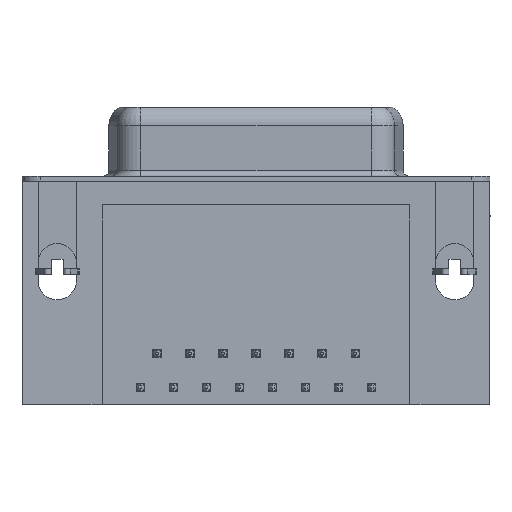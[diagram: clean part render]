
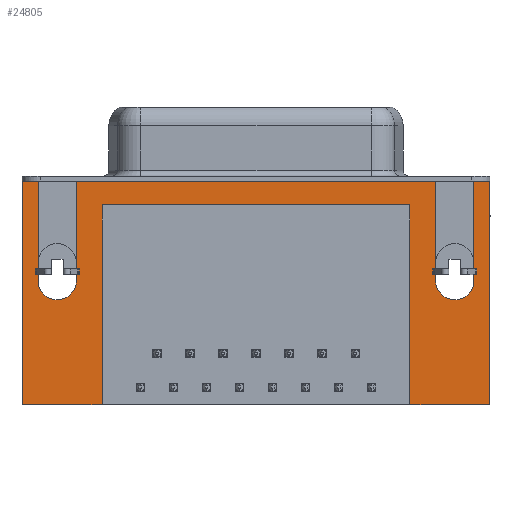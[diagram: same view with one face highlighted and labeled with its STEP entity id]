
A CAD part, front view. The second image highlights one B-rep face of the part: STEP entity #24805.
In plain terms, the highlighted planar face has unit normal (0, -1, 0).
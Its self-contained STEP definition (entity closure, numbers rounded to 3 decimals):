
#329 = CARTESIAN_POINT ( 'NONE',  ( -2.935, -6.275, 0. ) ) ;
#400 = VERTEX_POINT ( 'NONE', #22086 ) ;
#438 = ORIENTED_EDGE ( 'NONE', *, *, #1321, .F. ) ;
#682 = ORIENTED_EDGE ( 'NONE', *, *, #13333, .F. ) ;
#799 = CARTESIAN_POINT ( 'NONE',  ( -2.935, -6.275, 0. ) ) ;
#941 = FACE_OUTER_BOUND ( 'NONE', #15369, .T. ) ;
#1094 = CARTESIAN_POINT ( 'NONE',  ( 29.555, -6.275, -2. ) ) ;
#1101 = ORIENTED_EDGE ( 'NONE', *, *, #20498, .F. ) ;
#1321 = EDGE_CURVE ( 'NONE', #11784, #4898, #9651, .T. ) ;
#1620 = EDGE_CURVE ( 'NONE', #22914, #3859, #9228, .T. ) ;
#1792 = CARTESIAN_POINT ( 'NONE',  ( 3.765, -6.275, -2. ) ) ;
#1860 = DIRECTION ( 'NONE',  ( 0., 0., 1. ) ) ;
#2117 = DIRECTION ( 'NONE',  ( 0., 0., 1. ) ) ;
#2202 = DIRECTION ( 'NONE',  ( -1., 0., 0. ) ) ;
#2442 = CARTESIAN_POINT ( 'NONE',  ( 34.92, -6.275, 0. ) ) ;
#3032 = DIRECTION ( 'NONE',  ( 0., 0., -1. ) ) ;
#3361 = CARTESIAN_POINT ( 'NONE',  ( 31.72, -6.275, -8.35 ) ) ;
#3405 = DIRECTION ( 'NONE',  ( -1., 0., 0. ) ) ;
#3544 = EDGE_CURVE ( 'NONE', #16267, #22914, #26821, .T. ) ;
#3791 = CARTESIAN_POINT ( 'NONE',  ( 3.765, -6.275, -2. ) ) ;
#3859 = VERTEX_POINT ( 'NONE', #20307 ) ;
#3900 = DIRECTION ( 'NONE',  ( 0., 0., -1. ) ) ;
#4011 = CARTESIAN_POINT ( 'NONE',  ( 36.255, -6.275, -18.76 ) ) ;
#4176 = ORIENTED_EDGE ( 'NONE', *, *, #25894, .F. ) ;
#4520 = CARTESIAN_POINT ( 'NONE',  ( -1.6, -6.275, 0. ) ) ;
#4898 = VERTEX_POINT ( 'NONE', #5976 ) ;
#5200 = VERTEX_POINT ( 'NONE', #15408 ) ;
#5457 = EDGE_CURVE ( 'NONE', #5200, #16267, #13866, .T. ) ;
#5460 = VECTOR ( 'NONE', #7356, 1000. ) ;
#5506 = LINE ( 'NONE', #25995, #5460 ) ;
#5624 = ORIENTED_EDGE ( 'NONE', *, *, #1620, .F. ) ;
#5661 = VECTOR ( 'NONE', #3900, 1000. ) ;
#5976 = CARTESIAN_POINT ( 'NONE',  ( 1.6, -6.275, -8.35 ) ) ;
#6166 = CARTESIAN_POINT ( 'NONE',  ( 33.32, -6.275, -8.35 ) ) ;
#6206 = CARTESIAN_POINT ( 'NONE',  ( -2.935, -6.275, -2.5 ) ) ;
#6338 = VERTEX_POINT ( 'NONE', #4520 ) ;
#6771 = VECTOR ( 'NONE', #2117, 1000. ) ;
#6832 = EDGE_CURVE ( 'NONE', #4898, #24141, #6899, .T. ) ;
#6899 = LINE ( 'NONE', #18880, #6771 ) ;
#7152 = DIRECTION ( 'NONE',  ( 0., 0., 1. ) ) ;
#7177 = EDGE_CURVE ( 'NONE', #6338, #11784, #5506, .T. ) ;
#7356 = DIRECTION ( 'NONE',  ( 0., 0., -1. ) ) ;
#7525 = CARTESIAN_POINT ( 'NONE',  ( -2.935, -6.275, 0. ) ) ;
#7764 = CARTESIAN_POINT ( 'NONE',  ( -2.935, -6.275, -18.76 ) ) ;
#7915 = VECTOR ( 'NONE', #7152, 1000. ) ;
#8144 = ORIENTED_EDGE ( 'NONE', *, *, #9149, .F. ) ;
#8220 = LINE ( 'NONE', #11351, #7915 ) ;
#8268 = LINE ( 'NONE', #1792, #5661 ) ;
#8271 = DIRECTION ( 'NONE',  ( -1., 0., 0. ) ) ;
#8282 = ORIENTED_EDGE ( 'NONE', *, *, #5457, .F. ) ;
#8578 = VERTEX_POINT ( 'NONE', #12270 ) ;
#8662 = VERTEX_POINT ( 'NONE', #21041 ) ;
#8749 = VECTOR ( 'NONE', #1860, 1000. ) ;
#9149 = EDGE_CURVE ( 'NONE', #8662, #21470, #17370, .T. ) ;
#9228 = LINE ( 'NONE', #2442, #8749 ) ;
#9538 = VERTEX_POINT ( 'NONE', #4011 ) ;
#9651 = CIRCLE ( 'NONE', #10588, 1.6 ) ;
#9961 = ORIENTED_EDGE ( 'NONE', *, *, #7177, .F. ) ;
#10121 = ORIENTED_EDGE ( 'NONE', *, *, #11027, .F. ) ;
#10528 = EDGE_CURVE ( 'NONE', #16857, #8662, #8268, .T. ) ;
#10588 = AXIS2_PLACEMENT_3D ( 'NONE', #11688, #11680, #11626 ) ;
#11027 = EDGE_CURVE ( 'NONE', #8578, #16857, #26663, .T. ) ;
#11095 = EDGE_CURVE ( 'NONE', #3859, #400, #26489, .T. ) ;
#11351 = CARTESIAN_POINT ( 'NONE',  ( 36.255, -6.275, -2.5 ) ) ;
#11626 = DIRECTION ( 'NONE',  ( 1., 0., 0. ) ) ;
#11662 = VERTEX_POINT ( 'NONE', #25373 ) ;
#11680 = DIRECTION ( 'NONE',  ( 0., -1., 0. ) ) ;
#11688 = CARTESIAN_POINT ( 'NONE',  ( 0., -6.275, -8.35 ) ) ;
#11784 = VERTEX_POINT ( 'NONE', #17494 ) ;
#12270 = CARTESIAN_POINT ( 'NONE',  ( 29.555, -6.275, -2. ) ) ;
#12440 = EDGE_CURVE ( 'NONE', #11662, #8578, #22093, .T. ) ;
#12505 = DIRECTION ( 'NONE',  ( 0., 0., -1. ) ) ;
#13333 = EDGE_CURVE ( 'NONE', #9538, #11662, #19106, .T. ) ;
#13375 = CARTESIAN_POINT ( 'NONE',  ( -2.935, -6.275, -2.5 ) ) ;
#13434 = CARTESIAN_POINT ( 'NONE',  ( 31.72, -6.275, 0. ) ) ;
#13807 = CARTESIAN_POINT ( 'NONE',  ( 36.255, -6.275, -18.76 ) ) ;
#13818 = VECTOR ( 'NONE', #3032, 1000. ) ;
#13866 = LINE ( 'NONE', #13434, #13818 ) ;
#15044 = ORIENTED_EDGE ( 'NONE', *, *, #23292, .T. ) ;
#15369 = EDGE_LOOP ( 'NONE', ( #5624, #15910, #8282, #4176, #26650, #438, #9961, #1101, #17029, #8144, #24622, #10121, #17917, #682, #15044, #16400 ) ) ;
#15408 = CARTESIAN_POINT ( 'NONE',  ( 31.72, -6.275, 0. ) ) ;
#15526 = DIRECTION ( 'NONE',  ( 0., 0., 1. ) ) ;
#15910 = ORIENTED_EDGE ( 'NONE', *, *, #3544, .F. ) ;
#16267 = VERTEX_POINT ( 'NONE', #3361 ) ;
#16400 = ORIENTED_EDGE ( 'NONE', *, *, #11095, .F. ) ;
#16568 = AXIS2_PLACEMENT_3D ( 'NONE', #6206, #24995, #12505 ) ;
#16712 = PLANE ( 'NONE',  #16568 ) ;
#16857 = VERTEX_POINT ( 'NONE', #3791 ) ;
#16896 = CARTESIAN_POINT ( 'NONE',  ( 3.765, -6.275, -2. ) ) ;
#17029 = ORIENTED_EDGE ( 'NONE', *, *, #20937, .F. ) ;
#17370 = LINE ( 'NONE', #21455, #17443 ) ;
#17443 = VECTOR ( 'NONE', #23488, 1000. ) ;
#17487 = CARTESIAN_POINT ( 'NONE',  ( -2.935, -6.275, 0. ) ) ;
#17494 = CARTESIAN_POINT ( 'NONE',  ( -1.6, -6.275, -8.35 ) ) ;
#17917 = ORIENTED_EDGE ( 'NONE', *, *, #12440, .F. ) ;
#18880 = CARTESIAN_POINT ( 'NONE',  ( 1.6, -6.275, 0. ) ) ;
#18940 = VECTOR ( 'NONE', #15526, 1000. ) ;
#19092 = LINE ( 'NONE', #13375, #18940 ) ;
#19106 = LINE ( 'NONE', #13807, #19177 ) ;
#19177 = VECTOR ( 'NONE', #3405, 1000. ) ;
#19554 = DIRECTION ( 'NONE',  ( 1., 0., 0. ) ) ;
#20103 = DIRECTION ( 'NONE',  ( 0., 0., 1. ) ) ;
#20307 = CARTESIAN_POINT ( 'NONE',  ( 34.92, -6.275, 0. ) ) ;
#20498 = EDGE_CURVE ( 'NONE', #22673, #6338, #20707, .T. ) ;
#20539 = CARTESIAN_POINT ( 'NONE',  ( 34.92, -6.275, -8.35 ) ) ;
#20707 = LINE ( 'NONE', #7525, #20782 ) ;
#20782 = VECTOR ( 'NONE', #22244, 1000. ) ;
#20899 = DIRECTION ( 'NONE',  ( 0., -1., 0. ) ) ;
#20937 = EDGE_CURVE ( 'NONE', #21470, #22673, #19092, .T. ) ;
#21041 = CARTESIAN_POINT ( 'NONE',  ( 3.765, -6.275, -18.76 ) ) ;
#21455 = CARTESIAN_POINT ( 'NONE',  ( 36.255, -6.275, -18.76 ) ) ;
#21470 = VERTEX_POINT ( 'NONE', #7764 ) ;
#21570 = AXIS2_PLACEMENT_3D ( 'NONE', #6166, #20899, #8271 ) ;
#22086 = CARTESIAN_POINT ( 'NONE',  ( 36.255, -6.275, 0. ) ) ;
#22093 = LINE ( 'NONE', #1094, #22195 ) ;
#22195 = VECTOR ( 'NONE', #20103, 1000. ) ;
#22244 = DIRECTION ( 'NONE',  ( 1., 0., 0. ) ) ;
#22673 = VERTEX_POINT ( 'NONE', #799 ) ;
#22914 = VERTEX_POINT ( 'NONE', #20539 ) ;
#23077 = VECTOR ( 'NONE', #19554, 1000. ) ;
#23205 = LINE ( 'NONE', #17487, #23077 ) ;
#23292 = EDGE_CURVE ( 'NONE', #9538, #400, #8220, .T. ) ;
#23311 = DIRECTION ( 'NONE',  ( 1., 0., 0. ) ) ;
#23488 = DIRECTION ( 'NONE',  ( -1., 0., 0. ) ) ;
#24141 = VERTEX_POINT ( 'NONE', #26551 ) ;
#24622 = ORIENTED_EDGE ( 'NONE', *, *, #10528, .F. ) ;
#24805 = ADVANCED_FACE ( 'NONE', ( #941 ), #16712, .T. ) ;
#24995 = DIRECTION ( 'NONE',  ( 0., -1., 0. ) ) ;
#25373 = CARTESIAN_POINT ( 'NONE',  ( 29.555, -6.275, -18.76 ) ) ;
#25894 = EDGE_CURVE ( 'NONE', #24141, #5200, #23205, .T. ) ;
#25995 = CARTESIAN_POINT ( 'NONE',  ( -1.6, -6.275, 0. ) ) ;
#26355 = VECTOR ( 'NONE', #23311, 1000. ) ;
#26489 = LINE ( 'NONE', #329, #26355 ) ;
#26551 = CARTESIAN_POINT ( 'NONE',  ( 1.6, -6.275, 0. ) ) ;
#26650 = ORIENTED_EDGE ( 'NONE', *, *, #6832, .F. ) ;
#26663 = LINE ( 'NONE', #16896, #26732 ) ;
#26732 = VECTOR ( 'NONE', #2202, 1000. ) ;
#26821 = CIRCLE ( 'NONE', #21570, 1.6 ) ;
